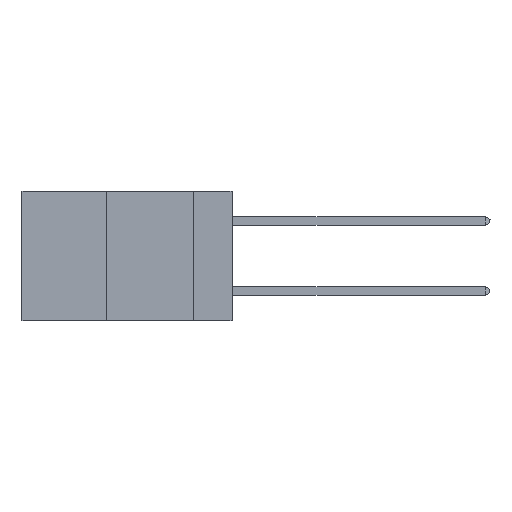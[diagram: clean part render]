
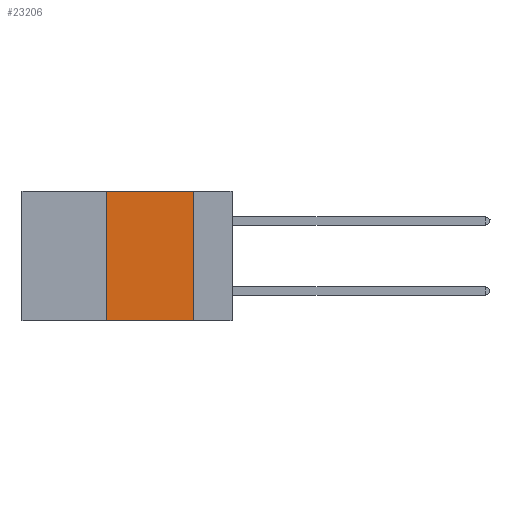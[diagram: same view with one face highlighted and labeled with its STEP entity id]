
A CAD part, left-side view. The second image highlights one B-rep face of the part: STEP entity #23206.
In plain terms, the highlighted planar face has unit normal (-1, 0, 0).
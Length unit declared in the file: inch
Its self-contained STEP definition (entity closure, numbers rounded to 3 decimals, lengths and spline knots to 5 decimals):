
#1225 = CARTESIAN_POINT ( 'NONE',  ( 0., 0.36, 0. ) ) ;
#1287 = CARTESIAN_POINT ( 'NONE',  ( 0., 0.11, 0. ) ) ;
#1439 = LINE ( 'NONE', #5158, #16161 ) ;
#1638 = VECTOR ( 'NONE', #23525, 39.37008 ) ;
#2837 = LINE ( 'NONE', #21885, #11760 ) ;
#3147 = PLANE ( 'NONE',  #20440 ) ;
#3683 = VERTEX_POINT ( 'NONE', #20626 ) ;
#4916 = CARTESIAN_POINT ( 'NONE',  ( 0., 0.36, 0. ) ) ;
#5158 = CARTESIAN_POINT ( 'NONE',  ( 0., 0.6, 0. ) ) ;
#6621 = LINE ( 'NONE', #1287, #8552 ) ;
#7234 = VERTEX_POINT ( 'NONE', #21920 ) ;
#7377 = VERTEX_POINT ( 'NONE', #1225 ) ;
#8552 = VECTOR ( 'NONE', #17733, 39.37008 ) ;
#8665 = EDGE_CURVE ( 'NONE', #7234, #7377, #21181, .T. ) ;
#9208 = DIRECTION ( 'NONE',  ( 0., -1., 0. ) ) ;
#9353 = DIRECTION ( 'NONE',  ( 1., 0., 0. ) ) ;
#10057 = VERTEX_POINT ( 'NONE', #15540 ) ;
#10976 = EDGE_LOOP ( 'NONE', ( #16950, #19909, #26430, #21037 ) ) ;
#11760 = VECTOR ( 'NONE', #9208, 39.37008 ) ;
#13286 = CARTESIAN_POINT ( 'NONE',  ( 0., 0.6, 0. ) ) ;
#14081 = EDGE_CURVE ( 'NONE', #7234, #10057, #2837, .T. ) ;
#15540 = CARTESIAN_POINT ( 'NONE',  ( 0., 0.11, -0.37 ) ) ;
#16161 = VECTOR ( 'NONE', #21853, 39.37008 ) ;
#16950 = ORIENTED_EDGE ( 'NONE', *, *, #20582, .F. ) ;
#17733 = DIRECTION ( 'NONE',  ( 0., 0., -1. ) ) ;
#19569 = FACE_OUTER_BOUND ( 'NONE', #10976, .T. ) ;
#19909 = ORIENTED_EDGE ( 'NONE', *, *, #21081, .F. ) ;
#20440 = AXIS2_PLACEMENT_3D ( 'NONE', #13286, #9353, #25567 ) ;
#20582 = EDGE_CURVE ( 'NONE', #3683, #10057, #6621, .T. ) ;
#20626 = CARTESIAN_POINT ( 'NONE',  ( 0., 0.11, 0. ) ) ;
#21037 = ORIENTED_EDGE ( 'NONE', *, *, #14081, .T. ) ;
#21081 = EDGE_CURVE ( 'NONE', #7377, #3683, #1439, .T. ) ;
#21181 = LINE ( 'NONE', #4916, #1638 ) ;
#21853 = DIRECTION ( 'NONE',  ( 0., -1., 0. ) ) ;
#21885 = CARTESIAN_POINT ( 'NONE',  ( 0., 0.6, -0.37 ) ) ;
#21920 = CARTESIAN_POINT ( 'NONE',  ( 0., 0.36, -0.37 ) ) ;
#23206 = ADVANCED_FACE ( 'NONE', ( #19569 ), #3147, .F. ) ;
#23525 = DIRECTION ( 'NONE',  ( 0., 0., 1. ) ) ;
#25567 = DIRECTION ( 'NONE',  ( 0., 0., -1. ) ) ;
#26430 = ORIENTED_EDGE ( 'NONE', *, *, #8665, .F. ) ;
